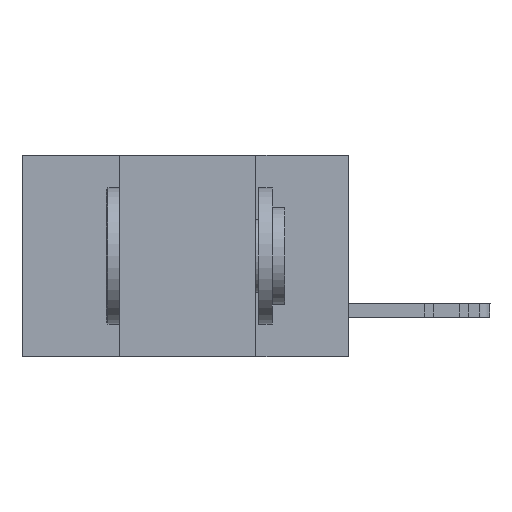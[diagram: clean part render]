
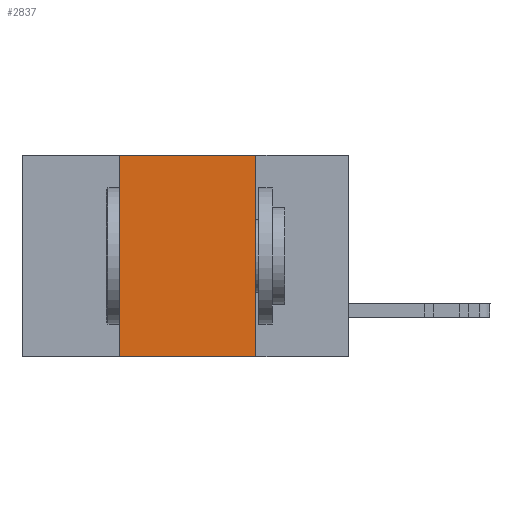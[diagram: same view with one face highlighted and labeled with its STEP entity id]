
A CAD part, left-side view. The second image highlights one B-rep face of the part: STEP entity #2837.
In plain terms, the highlighted planar face has unit normal (-1, 0, 0).
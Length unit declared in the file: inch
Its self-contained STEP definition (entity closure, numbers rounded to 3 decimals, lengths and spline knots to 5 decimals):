
#951 = CARTESIAN_POINT ( 'NONE',  ( 0., 0.42, 0. ) ) ;
#1663 = LINE ( 'NONE', #8975, #17639 ) ;
#1945 = FACE_OUTER_BOUND ( 'NONE', #19791, .T. ) ;
#2688 = EDGE_CURVE ( 'NONE', #20964, #12895, #24236, .T. ) ;
#2766 = VERTEX_POINT ( 'NONE', #10863 ) ;
#2837 = ADVANCED_FACE ( 'NONE', ( #1945 ), #3806, .F. ) ;
#3407 = AXIS2_PLACEMENT_3D ( 'NONE', #11375, #23996, #9010 ) ;
#3806 = PLANE ( 'NONE',  #3407 ) ;
#4682 = EDGE_CURVE ( 'NONE', #8823, #2766, #6006, .T. ) ;
#5418 = ORIENTED_EDGE ( 'NONE', *, *, #2688, .T. ) ;
#6006 = LINE ( 'NONE', #13801, #13363 ) ;
#8438 = ORIENTED_EDGE ( 'NONE', *, *, #20668, .F. ) ;
#8823 = VERTEX_POINT ( 'NONE', #951 ) ;
#8975 = CARTESIAN_POINT ( 'NONE',  ( 0., 0.42, -0.37 ) ) ;
#9010 = DIRECTION ( 'NONE',  ( 0., 0., -1. ) ) ;
#10863 = CARTESIAN_POINT ( 'NONE',  ( 0., 0.17, 0. ) ) ;
#10928 = CARTESIAN_POINT ( 'NONE',  ( 0., 0.17, -0.37 ) ) ;
#11375 = CARTESIAN_POINT ( 'NONE',  ( 0., 0.6, 0. ) ) ;
#12367 = EDGE_CURVE ( 'NONE', #20964, #8823, #1663, .T. ) ;
#12895 = VERTEX_POINT ( 'NONE', #10928 ) ;
#12941 = ORIENTED_EDGE ( 'NONE', *, *, #12367, .F. ) ;
#13363 = VECTOR ( 'NONE', #21110, 39.37008 ) ;
#13801 = CARTESIAN_POINT ( 'NONE',  ( 0., 0.6, 0. ) ) ;
#14671 = DIRECTION ( 'NONE',  ( 0., 0., 1. ) ) ;
#14876 = VECTOR ( 'NONE', #16430, 39.37008 ) ;
#15312 = ORIENTED_EDGE ( 'NONE', *, *, #4682, .F. ) ;
#16430 = DIRECTION ( 'NONE',  ( 0., -1., 0. ) ) ;
#16678 = CARTESIAN_POINT ( 'NONE',  ( 0., 0.6, -0.37 ) ) ;
#17639 = VECTOR ( 'NONE', #14671, 39.37008 ) ;
#18949 = CARTESIAN_POINT ( 'NONE',  ( 0., 0.42, -0.37 ) ) ;
#19578 = CARTESIAN_POINT ( 'NONE',  ( 0., 0.17, -0.37 ) ) ;
#19699 = LINE ( 'NONE', #19578, #23347 ) ;
#19791 = EDGE_LOOP ( 'NONE', ( #8438, #15312, #12941, #5418 ) ) ;
#20668 = EDGE_CURVE ( 'NONE', #2766, #12895, #19699, .T. ) ;
#20964 = VERTEX_POINT ( 'NONE', #18949 ) ;
#21110 = DIRECTION ( 'NONE',  ( 0., -1., 0. ) ) ;
#23300 = DIRECTION ( 'NONE',  ( 0., 0., -1. ) ) ;
#23347 = VECTOR ( 'NONE', #23300, 39.37008 ) ;
#23996 = DIRECTION ( 'NONE',  ( 1., 0., 0. ) ) ;
#24236 = LINE ( 'NONE', #16678, #14876 ) ;
